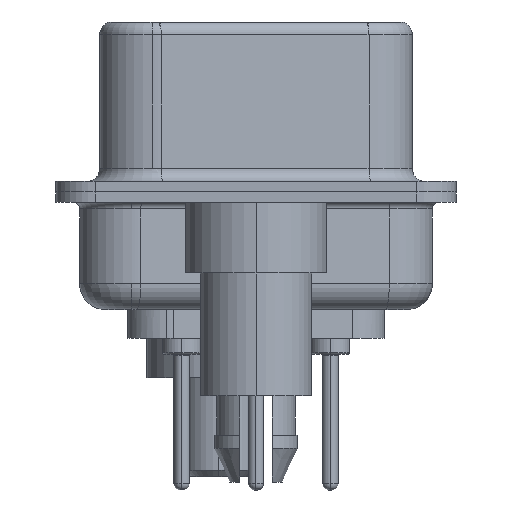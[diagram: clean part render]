
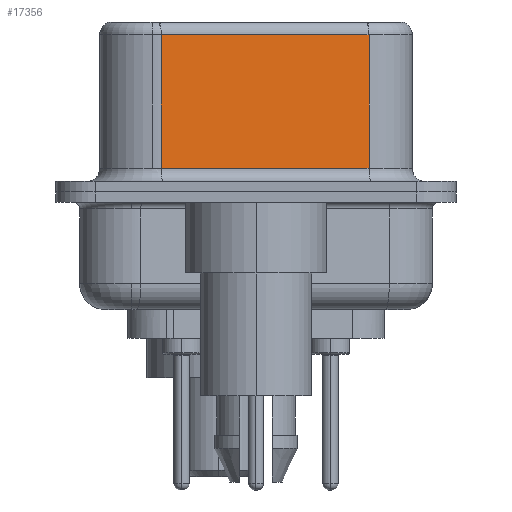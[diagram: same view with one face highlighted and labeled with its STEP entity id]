
A CAD part, left-side view. The second image highlights one B-rep face of the part: STEP entity #17356.
In plain terms, the highlighted planar face has unit normal (-0.985, -0.174, 0).
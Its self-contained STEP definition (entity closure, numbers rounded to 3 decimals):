
#1145 = CARTESIAN_POINT ( 'NONE',  ( 3.73, 3.628, 6.52 ) ) ;
#3135 = DIRECTION ( 'NONE',  ( 0., 0., -1. ) ) ;
#4246 = ORIENTED_EDGE ( 'NONE', *, *, #29776, .T. ) ;
#6348 = VERTEX_POINT ( 'NONE', #11685 ) ;
#7356 = VERTEX_POINT ( 'NONE', #33941 ) ;
#9339 = LINE ( 'NONE', #11504, #29350 ) ;
#11202 = VERTEX_POINT ( 'NONE', #34312 ) ;
#11504 = CARTESIAN_POINT ( 'NONE',  ( 5.132, -4.322, 6.52 ) ) ;
#11685 = CARTESIAN_POINT ( 'NONE',  ( 5.132, -4.322, 0.9 ) ) ;
#14075 = DIRECTION ( 'NONE',  ( 0., 0., -1. ) ) ;
#15804 = DIRECTION ( 'NONE',  ( 0.174, -0.985, 0. ) ) ;
#16190 = EDGE_LOOP ( 'NONE', ( #33602, #4246, #23065, #16331 ) ) ;
#16331 = ORIENTED_EDGE ( 'NONE', *, *, #16474, .T. ) ;
#16474 = EDGE_CURVE ( 'NONE', #7356, #6348, #23452, .T. ) ;
#16539 = AXIS2_PLACEMENT_3D ( 'NONE', #25721, #25614, #33666 ) ;
#17356 = ADVANCED_FACE ( 'NONE', ( #30047 ), #22713, .F. ) ;
#17582 = LINE ( 'NONE', #26957, #26313 ) ;
#17907 = EDGE_CURVE ( 'NONE', #11202, #6348, #9339, .T. ) ;
#17939 = VERTEX_POINT ( 'NONE', #32824 ) ;
#18868 = EDGE_CURVE ( 'NONE', #17939, #7356, #27185, .T. ) ;
#20700 = CARTESIAN_POINT ( 'NONE',  ( 5.132, -4.322, 0.9 ) ) ;
#22172 = VECTOR ( 'NONE', #14075, 1000. ) ;
#22713 = PLANE ( 'NONE',  #16539 ) ;
#23065 = ORIENTED_EDGE ( 'NONE', *, *, #18868, .T. ) ;
#23452 = LINE ( 'NONE', #20700, #28048 ) ;
#24139 = DIRECTION ( 'NONE',  ( -0.174, 0.985, 0. ) ) ;
#25614 = DIRECTION ( 'NONE',  ( 0.985, 0.174, 0. ) ) ;
#25721 = CARTESIAN_POINT ( 'NONE',  ( 5.132, -4.322, 6.52 ) ) ;
#26313 = VECTOR ( 'NONE', #24139, 1000. ) ;
#26957 = CARTESIAN_POINT ( 'NONE',  ( 5.132, -4.322, 6.02 ) ) ;
#27185 = LINE ( 'NONE', #1145, #22172 ) ;
#28048 = VECTOR ( 'NONE', #15804, 1000. ) ;
#29350 = VECTOR ( 'NONE', #3135, 1000. ) ;
#29776 = EDGE_CURVE ( 'NONE', #11202, #17939, #17582, .T. ) ;
#30047 = FACE_OUTER_BOUND ( 'NONE', #16190, .T. ) ;
#32824 = CARTESIAN_POINT ( 'NONE',  ( 3.73, 3.628, 6.02 ) ) ;
#33602 = ORIENTED_EDGE ( 'NONE', *, *, #17907, .F. ) ;
#33666 = DIRECTION ( 'NONE',  ( -0.174, 0.985, 0. ) ) ;
#33941 = CARTESIAN_POINT ( 'NONE',  ( 3.73, 3.628, 0.9 ) ) ;
#34312 = CARTESIAN_POINT ( 'NONE',  ( 5.132, -4.322, 6.02 ) ) ;
